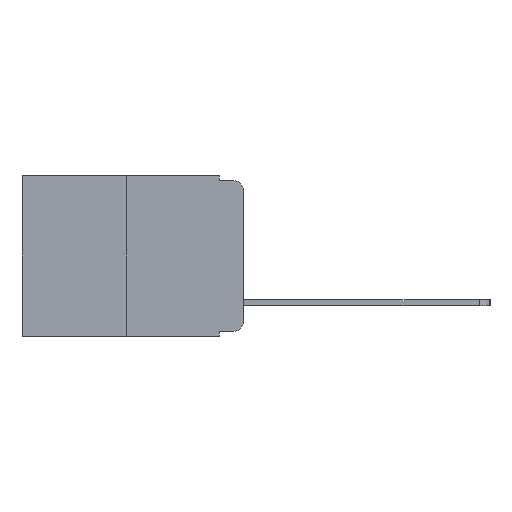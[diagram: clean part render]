
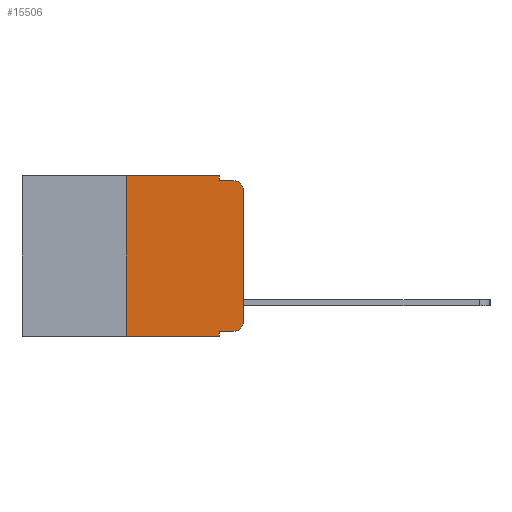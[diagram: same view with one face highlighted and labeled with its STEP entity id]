
A CAD part, left-side view. The second image highlights one B-rep face of the part: STEP entity #15506.
In plain terms, the highlighted planar face has unit normal (-1, 0, 0).
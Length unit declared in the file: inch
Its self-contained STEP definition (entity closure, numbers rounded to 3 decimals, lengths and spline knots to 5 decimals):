
#103 = EDGE_CURVE ( 'NONE', #9661, #8161, #10864, .T. ) ;
#183 = DIRECTION ( 'NONE',  ( 0., -1., 0. ) ) ;
#197 = CARTESIAN_POINT ( 'NONE',  ( 0., 0.473, 0. ) ) ;
#811 = CARTESIAN_POINT ( 'NONE',  ( 0., 0.25, 0. ) ) ;
#1163 = VERTEX_POINT ( 'NONE', #15639 ) ;
#1197 = LINE ( 'NONE', #14281, #5139 ) ;
#1301 = ORIENTED_EDGE ( 'NONE', *, *, #17583, .F. ) ;
#1647 = EDGE_CURVE ( 'NONE', #16682, #9661, #9937, .T. ) ;
#1878 = CARTESIAN_POINT ( 'NONE',  ( 0., 0.051, -0.343 ) ) ;
#2039 = VERTEX_POINT ( 'NONE', #8373 ) ;
#2476 = AXIS2_PLACEMENT_3D ( 'NONE', #15725, #7686, #17035 ) ;
#2701 = DIRECTION ( 'NONE',  ( 0., 0., -1. ) ) ;
#2806 = AXIS2_PLACEMENT_3D ( 'NONE', #5352, #14848, #6746 ) ;
#3160 = ORIENTED_EDGE ( 'NONE', *, *, #1647, .F. ) ;
#3263 = LINE ( 'NONE', #4120, #6652 ) ;
#3486 = VECTOR ( 'NONE', #183, 39.37008 ) ;
#3604 = ORIENTED_EDGE ( 'NONE', *, *, #8599, .T. ) ;
#3727 = VERTEX_POINT ( 'NONE', #1878 ) ;
#3774 = CARTESIAN_POINT ( 'NONE',  ( 0., 0.051, 0. ) ) ;
#3787 = EDGE_CURVE ( 'NONE', #2039, #1163, #12497, .T. ) ;
#4042 = ORIENTED_EDGE ( 'NONE', *, *, #13675, .F. ) ;
#4120 = CARTESIAN_POINT ( 'NONE',  ( 0., 0.051, -0.01 ) ) ;
#4263 = CARTESIAN_POINT ( 'NONE',  ( 0., 0.051, 0. ) ) ;
#4600 = CIRCLE ( 'NONE', #2476, 0.02 ) ;
#4702 = DIRECTION ( 'NONE',  ( 0., -1., 0. ) ) ;
#5139 = VECTOR ( 'NONE', #4702, 39.37008 ) ;
#5265 = DIRECTION ( 'NONE',  ( 0., 0., 1. ) ) ;
#5352 = CARTESIAN_POINT ( 'NONE',  ( 0., 0.02, -0.03 ) ) ;
#5601 = EDGE_CURVE ( 'NONE', #16133, #13866, #1197, .T. ) ;
#5602 = VECTOR ( 'NONE', #5265, 39.37008 ) ;
#6100 = CARTESIAN_POINT ( 'NONE',  ( 0., 0.02, -0.333 ) ) ;
#6208 = VECTOR ( 'NONE', #2701, 39.37008 ) ;
#6558 = DIRECTION ( 'NONE',  ( 0., 0., -1. ) ) ;
#6652 = VECTOR ( 'NONE', #11090, 39.37008 ) ;
#6731 = VECTOR ( 'NONE', #10197, 39.37008 ) ;
#6746 = DIRECTION ( 'NONE',  ( 0., 0., -1. ) ) ;
#6999 = EDGE_CURVE ( 'NONE', #13866, #2039, #4600, .T. ) ;
#7173 = CARTESIAN_POINT ( 'NONE',  ( 0., 0.051, -0.333 ) ) ;
#7395 = EDGE_LOOP ( 'NONE', ( #11695, #12120, #1301, #16416, #3160, #10628, #3604, #4042, #11493, #13983 ) ) ;
#7686 = DIRECTION ( 'NONE',  ( -1., 0., 0. ) ) ;
#7872 = PLANE ( 'NONE',  #14060 ) ;
#8123 = CARTESIAN_POINT ( 'NONE',  ( 0., 0.25, 0. ) ) ;
#8161 = VERTEX_POINT ( 'NONE', #15900 ) ;
#8373 = CARTESIAN_POINT ( 'NONE',  ( 0., 0., -0.313 ) ) ;
#8552 = CARTESIAN_POINT ( 'NONE',  ( 0., 0.02, -0.01 ) ) ;
#8599 = EDGE_CURVE ( 'NONE', #12307, #3727, #14909, .T. ) ;
#9059 = CIRCLE ( 'NONE', #2806, 0.02 ) ;
#9148 = VERTEX_POINT ( 'NONE', #8552 ) ;
#9279 = LINE ( 'NONE', #811, #5602 ) ;
#9661 = VERTEX_POINT ( 'NONE', #4263 ) ;
#9832 = LINE ( 'NONE', #12484, #6208 ) ;
#9937 = LINE ( 'NONE', #197, #6731 ) ;
#10197 = DIRECTION ( 'NONE',  ( 0., -1., 0. ) ) ;
#10217 = DIRECTION ( 'NONE',  ( 0., 0., -1. ) ) ;
#10460 = DIRECTION ( 'NONE',  ( 0., 0., 1. ) ) ;
#10624 = CARTESIAN_POINT ( 'NONE',  ( 0., 0.473, 0. ) ) ;
#10628 = ORIENTED_EDGE ( 'NONE', *, *, #11451, .F. ) ;
#10864 = LINE ( 'NONE', #3774, #17073 ) ;
#11090 = DIRECTION ( 'NONE',  ( 0., -1., 0. ) ) ;
#11451 = EDGE_CURVE ( 'NONE', #12307, #16682, #9279, .T. ) ;
#11493 = ORIENTED_EDGE ( 'NONE', *, *, #5601, .T. ) ;
#11695 = ORIENTED_EDGE ( 'NONE', *, *, #3787, .T. ) ;
#12120 = ORIENTED_EDGE ( 'NONE', *, *, #16672, .T. ) ;
#12307 = VERTEX_POINT ( 'NONE', #13988 ) ;
#12484 = CARTESIAN_POINT ( 'NONE',  ( 0., 0.051, 0. ) ) ;
#12497 = LINE ( 'NONE', #14506, #16388 ) ;
#13675 = EDGE_CURVE ( 'NONE', #16133, #3727, #9832, .T. ) ;
#13866 = VERTEX_POINT ( 'NONE', #6100 ) ;
#13983 = ORIENTED_EDGE ( 'NONE', *, *, #6999, .T. ) ;
#13988 = CARTESIAN_POINT ( 'NONE',  ( 0., 0.25, -0.343 ) ) ;
#14060 = AXIS2_PLACEMENT_3D ( 'NONE', #10624, #14658, #6558 ) ;
#14281 = CARTESIAN_POINT ( 'NONE',  ( 0., 0.051, -0.333 ) ) ;
#14506 = CARTESIAN_POINT ( 'NONE',  ( 0., 0., 0. ) ) ;
#14658 = DIRECTION ( 'NONE',  ( 1., 0., 0. ) ) ;
#14848 = DIRECTION ( 'NONE',  ( -1., 0., 0. ) ) ;
#14909 = LINE ( 'NONE', #15482, #3486 ) ;
#15482 = CARTESIAN_POINT ( 'NONE',  ( 0., 0.473, -0.343 ) ) ;
#15506 = ADVANCED_FACE ( 'NONE', ( #17800 ), #7872, .F. ) ;
#15639 = CARTESIAN_POINT ( 'NONE',  ( 0., 0., -0.03 ) ) ;
#15725 = CARTESIAN_POINT ( 'NONE',  ( 0., 0.02, -0.313 ) ) ;
#15900 = CARTESIAN_POINT ( 'NONE',  ( 0., 0.051, -0.01 ) ) ;
#16133 = VERTEX_POINT ( 'NONE', #7173 ) ;
#16388 = VECTOR ( 'NONE', #10460, 39.37008 ) ;
#16416 = ORIENTED_EDGE ( 'NONE', *, *, #103, .F. ) ;
#16672 = EDGE_CURVE ( 'NONE', #1163, #9148, #9059, .T. ) ;
#16682 = VERTEX_POINT ( 'NONE', #8123 ) ;
#17035 = DIRECTION ( 'NONE',  ( 0., 0., -1. ) ) ;
#17073 = VECTOR ( 'NONE', #10217, 39.37008 ) ;
#17583 = EDGE_CURVE ( 'NONE', #8161, #9148, #3263, .T. ) ;
#17800 = FACE_OUTER_BOUND ( 'NONE', #7395, .T. ) ;
